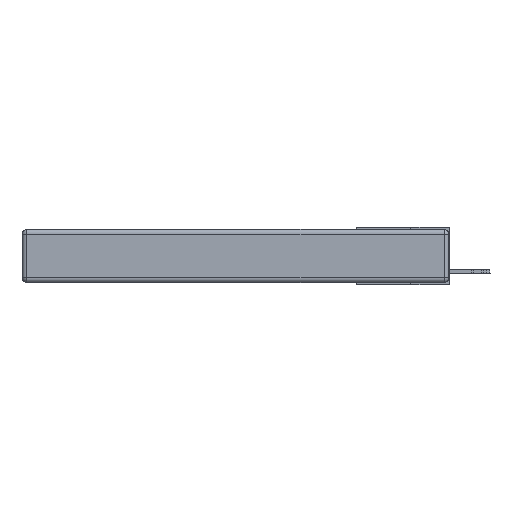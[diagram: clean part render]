
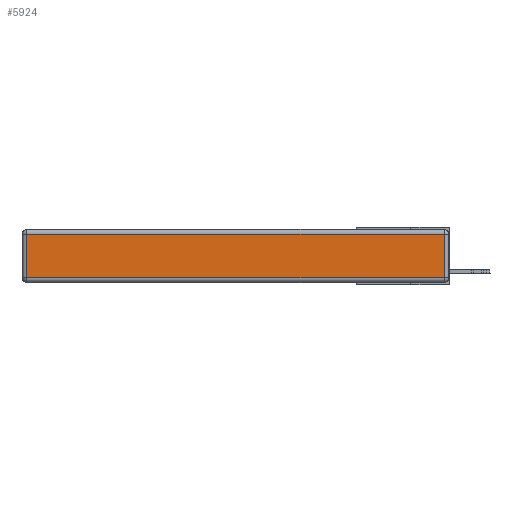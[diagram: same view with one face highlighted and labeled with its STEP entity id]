
A CAD part, left-side view. The second image highlights one B-rep face of the part: STEP entity #5924.
In plain terms, the highlighted planar face has unit normal (-1, 0, 0).
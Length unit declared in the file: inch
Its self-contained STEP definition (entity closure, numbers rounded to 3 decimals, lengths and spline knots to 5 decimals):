
#692 = DIRECTION ( 'NONE',  ( 0., 0., 1. ) ) ;
#693 = LINE ( 'NONE', #25308, #25730 ) ;
#1950 = VECTOR ( 'NONE', #692, 39.37008 ) ;
#2006 = VERTEX_POINT ( 'NONE', #19645 ) ;
#3998 = CARTESIAN_POINT ( 'NONE',  ( 0., 0., -0.343 ) ) ;
#5034 = LINE ( 'NONE', #30196, #1950 ) ;
#5924 = ADVANCED_FACE ( 'NONE', ( #10263 ), #25263, .T. ) ;
#7343 = EDGE_CURVE ( 'NONE', #29713, #24160, #693, .T. ) ;
#7658 = CARTESIAN_POINT ( 'NONE',  ( 0., 0.03, -0.03 ) ) ;
#8128 = EDGE_CURVE ( 'NONE', #2006, #25229, #5034, .T. ) ;
#9904 = CARTESIAN_POINT ( 'NONE',  ( 0., 2.72, -0.313 ) ) ;
#10084 = CARTESIAN_POINT ( 'NONE',  ( 0., 0., -0.313 ) ) ;
#10263 = FACE_OUTER_BOUND ( 'NONE', #12531, .T. ) ;
#10591 = AXIS2_PLACEMENT_3D ( 'NONE', #3998, #20614, #25483 ) ;
#12531 = EDGE_LOOP ( 'NONE', ( #21553, #30033, #19569, #28820 ) ) ;
#12547 = VECTOR ( 'NONE', #27114, 39.37008 ) ;
#15069 = DIRECTION ( 'NONE',  ( 0., -1., 0. ) ) ;
#17846 = EDGE_CURVE ( 'NONE', #25229, #29713, #18238, .T. ) ;
#18238 = LINE ( 'NONE', #19576, #12547 ) ;
#19530 = CARTESIAN_POINT ( 'NONE',  ( 0., 2.72, -0.03 ) ) ;
#19569 = ORIENTED_EDGE ( 'NONE', *, *, #17846, .T. ) ;
#19576 = CARTESIAN_POINT ( 'NONE',  ( 0., 2.75, -0.03 ) ) ;
#19645 = CARTESIAN_POINT ( 'NONE',  ( 0., 0.03, -0.313 ) ) ;
#20614 = DIRECTION ( 'NONE',  ( -1., 0., 0. ) ) ;
#21553 = ORIENTED_EDGE ( 'NONE', *, *, #31055, .T. ) ;
#23192 = VECTOR ( 'NONE', #15069, 39.37008 ) ;
#23933 = LINE ( 'NONE', #10084, #23192 ) ;
#24160 = VERTEX_POINT ( 'NONE', #9904 ) ;
#25229 = VERTEX_POINT ( 'NONE', #7658 ) ;
#25263 = PLANE ( 'NONE',  #10591 ) ;
#25308 = CARTESIAN_POINT ( 'NONE',  ( 0., 2.72, -0.343 ) ) ;
#25483 = DIRECTION ( 'NONE',  ( 0., 0., 1. ) ) ;
#25730 = VECTOR ( 'NONE', #27776, 39.37008 ) ;
#27114 = DIRECTION ( 'NONE',  ( 0., 1., 0. ) ) ;
#27776 = DIRECTION ( 'NONE',  ( 0., 0., -1. ) ) ;
#28820 = ORIENTED_EDGE ( 'NONE', *, *, #7343, .T. ) ;
#29713 = VERTEX_POINT ( 'NONE', #19530 ) ;
#30033 = ORIENTED_EDGE ( 'NONE', *, *, #8128, .T. ) ;
#30196 = CARTESIAN_POINT ( 'NONE',  ( 0., 0.03, -0.343 ) ) ;
#31055 = EDGE_CURVE ( 'NONE', #24160, #2006, #23933, .T. ) ;
